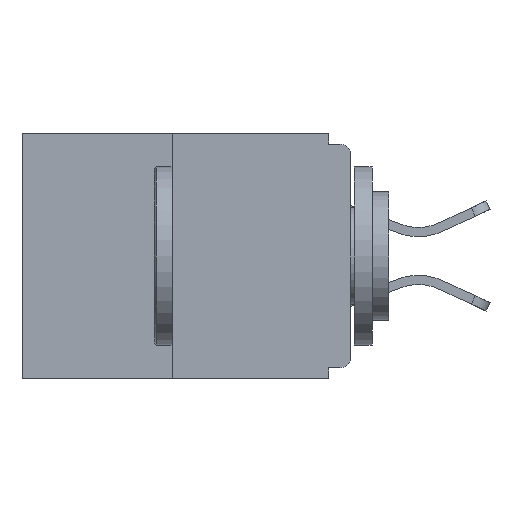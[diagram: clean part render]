
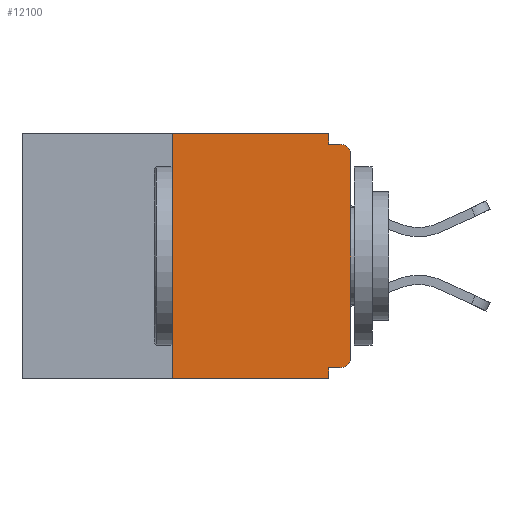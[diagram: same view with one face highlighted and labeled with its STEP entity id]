
A CAD part, left-side view. The second image highlights one B-rep face of the part: STEP entity #12100.
In plain terms, the highlighted planar face has unit normal (-1, 0, 0).
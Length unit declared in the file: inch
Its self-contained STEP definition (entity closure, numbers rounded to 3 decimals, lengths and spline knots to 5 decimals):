
#719 = PLANE ( 'NONE',  #26726 ) ;
#1103 = EDGE_CURVE ( 'NONE', #18797, #28568, #24972, .T. ) ;
#1738 = CARTESIAN_POINT ( 'NONE',  ( 0., 0.25, 0. ) ) ;
#2005 = LINE ( 'NONE', #17103, #20001 ) ;
#2063 = ORIENTED_EDGE ( 'NONE', *, *, #23790, .F. ) ;
#2247 = CARTESIAN_POINT ( 'NONE',  ( 0., 0.031, -0.015 ) ) ;
#2467 = CARTESIAN_POINT ( 'NONE',  ( 0., 0.46, 0. ) ) ;
#2527 = CARTESIAN_POINT ( 'NONE',  ( 0., 0.46, -0.343 ) ) ;
#2702 = EDGE_CURVE ( 'NONE', #15948, #20107, #8315, .T. ) ;
#2719 = ORIENTED_EDGE ( 'NONE', *, *, #5456, .T. ) ;
#3036 = DIRECTION ( 'NONE',  ( 0., 0., -1. ) ) ;
#3148 = CARTESIAN_POINT ( 'NONE',  ( 0., 0.46, 0. ) ) ;
#3259 = CIRCLE ( 'NONE', #14725, 0.015 ) ;
#3483 = ORIENTED_EDGE ( 'NONE', *, *, #7097, .F. ) ;
#3566 = VERTEX_POINT ( 'NONE', #1738 ) ;
#3868 = EDGE_CURVE ( 'NONE', #14076, #20469, #25793, .T. ) ;
#4371 = VECTOR ( 'NONE', #21532, 39.37008 ) ;
#4769 = VECTOR ( 'NONE', #15269, 39.37008 ) ;
#4793 = CARTESIAN_POINT ( 'NONE',  ( 0., 0., -0.328 ) ) ;
#4813 = CARTESIAN_POINT ( 'NONE',  ( 0., 0.015, -0.313 ) ) ;
#5456 = EDGE_CURVE ( 'NONE', #18935, #15948, #20565, .T. ) ;
#5845 = ORIENTED_EDGE ( 'NONE', *, *, #20987, .T. ) ;
#5997 = CARTESIAN_POINT ( 'NONE',  ( 0., 0.031, -0.343 ) ) ;
#6109 = LINE ( 'NONE', #6645, #8674 ) ;
#6370 = ORIENTED_EDGE ( 'NONE', *, *, #23524, .F. ) ;
#6645 = CARTESIAN_POINT ( 'NONE',  ( 0., 0.25, 0. ) ) ;
#6670 = AXIS2_PLACEMENT_3D ( 'NONE', #27164, #22467, #13084 ) ;
#6951 = VERTEX_POINT ( 'NONE', #14968 ) ;
#7097 = EDGE_CURVE ( 'NONE', #6951, #26021, #23793, .T. ) ;
#7203 = CARTESIAN_POINT ( 'NONE',  ( 0., 0., -0.313 ) ) ;
#7348 = DIRECTION ( 'NONE',  ( 0., -1., 0. ) ) ;
#7609 = VECTOR ( 'NONE', #16324, 39.37008 ) ;
#8175 = CARTESIAN_POINT ( 'NONE',  ( 0., 0., 0. ) ) ;
#8315 = CIRCLE ( 'NONE', #6670, 0.015 ) ;
#8674 = VECTOR ( 'NONE', #18365, 39.37008 ) ;
#9523 = DIRECTION ( 'NONE',  ( -1., 0., 0. ) ) ;
#10198 = LINE ( 'NONE', #2467, #7609 ) ;
#12100 = ADVANCED_FACE ( 'NONE', ( #20501 ), #719, .F. ) ;
#12173 = DIRECTION ( 'NONE',  ( 1., 0., 0. ) ) ;
#12963 = DIRECTION ( 'NONE',  ( 0., -1., 0. ) ) ;
#13084 = DIRECTION ( 'NONE',  ( 0., 0., -1. ) ) ;
#13611 = ORIENTED_EDGE ( 'NONE', *, *, #1103, .F. ) ;
#14076 = VERTEX_POINT ( 'NONE', #19295 ) ;
#14725 = AXIS2_PLACEMENT_3D ( 'NONE', #4813, #9523, #23822 ) ;
#14744 = CARTESIAN_POINT ( 'NONE',  ( 0., 0.015, -0.015 ) ) ;
#14837 = EDGE_CURVE ( 'NONE', #26021, #20107, #16247, .T. ) ;
#14968 = CARTESIAN_POINT ( 'NONE',  ( 0., 0.031, 0. ) ) ;
#15208 = ORIENTED_EDGE ( 'NONE', *, *, #3868, .T. ) ;
#15269 = DIRECTION ( 'NONE',  ( 0., 0., 1. ) ) ;
#15948 = VERTEX_POINT ( 'NONE', #17013 ) ;
#16247 = LINE ( 'NONE', #29109, #22857 ) ;
#16324 = DIRECTION ( 'NONE',  ( 0., -1., 0. ) ) ;
#17013 = CARTESIAN_POINT ( 'NONE',  ( 0., 0., -0.03 ) ) ;
#17103 = CARTESIAN_POINT ( 'NONE',  ( 0., 0.031, -0.343 ) ) ;
#17511 = VECTOR ( 'NONE', #29891, 39.37008 ) ;
#18213 = CARTESIAN_POINT ( 'NONE',  ( 0., 0.015, -0.328 ) ) ;
#18365 = DIRECTION ( 'NONE',  ( 0., 0., 1. ) ) ;
#18797 = VERTEX_POINT ( 'NONE', #18213 ) ;
#18935 = VERTEX_POINT ( 'NONE', #7203 ) ;
#19295 = CARTESIAN_POINT ( 'NONE',  ( 0., 0.25, -0.343 ) ) ;
#20001 = VECTOR ( 'NONE', #3036, 39.37008 ) ;
#20107 = VERTEX_POINT ( 'NONE', #14744 ) ;
#20169 = ORIENTED_EDGE ( 'NONE', *, *, #25253, .F. ) ;
#20469 = VERTEX_POINT ( 'NONE', #5997 ) ;
#20501 = FACE_OUTER_BOUND ( 'NONE', #26236, .T. ) ;
#20565 = LINE ( 'NONE', #8175, #4769 ) ;
#20987 = EDGE_CURVE ( 'NONE', #18797, #18935, #3259, .T. ) ;
#21532 = DIRECTION ( 'NONE',  ( 0., 1., 0. ) ) ;
#22383 = ORIENTED_EDGE ( 'NONE', *, *, #2702, .T. ) ;
#22467 = DIRECTION ( 'NONE',  ( -1., 0., 0. ) ) ;
#22857 = VECTOR ( 'NONE', #12963, 39.37008 ) ;
#22984 = CARTESIAN_POINT ( 'NONE',  ( 0., 0.031, -0.328 ) ) ;
#23524 = EDGE_CURVE ( 'NONE', #3566, #6951, #10198, .T. ) ;
#23790 = EDGE_CURVE ( 'NONE', #14076, #3566, #6109, .T. ) ;
#23793 = LINE ( 'NONE', #27106, #17511 ) ;
#23822 = DIRECTION ( 'NONE',  ( 0., 0., -1. ) ) ;
#24972 = LINE ( 'NONE', #4793, #4371 ) ;
#25253 = EDGE_CURVE ( 'NONE', #28568, #20469, #2005, .T. ) ;
#25793 = LINE ( 'NONE', #2527, #28008 ) ;
#26021 = VERTEX_POINT ( 'NONE', #2247 ) ;
#26073 = ORIENTED_EDGE ( 'NONE', *, *, #14837, .F. ) ;
#26236 = EDGE_LOOP ( 'NONE', ( #6370, #2063, #15208, #20169, #13611, #5845, #2719, #22383, #26073, #3483 ) ) ;
#26648 = DIRECTION ( 'NONE',  ( 0., 0., -1. ) ) ;
#26726 = AXIS2_PLACEMENT_3D ( 'NONE', #3148, #12173, #26648 ) ;
#27106 = CARTESIAN_POINT ( 'NONE',  ( 0., 0.031, 0. ) ) ;
#27164 = CARTESIAN_POINT ( 'NONE',  ( 0., 0.015, -0.03 ) ) ;
#28008 = VECTOR ( 'NONE', #7348, 39.37008 ) ;
#28568 = VERTEX_POINT ( 'NONE', #22984 ) ;
#29109 = CARTESIAN_POINT ( 'NONE',  ( 0., 0., -0.015 ) ) ;
#29891 = DIRECTION ( 'NONE',  ( 0., 0., -1. ) ) ;
